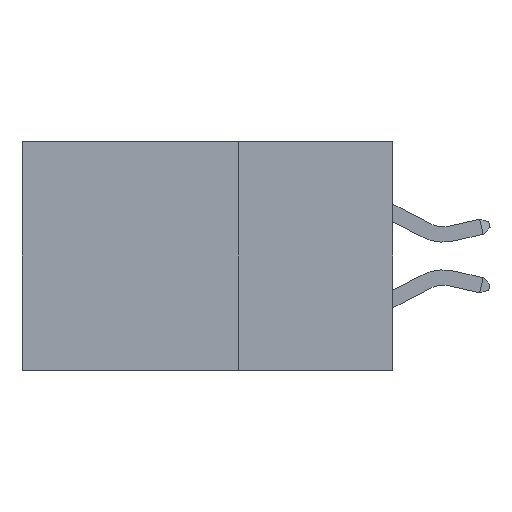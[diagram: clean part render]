
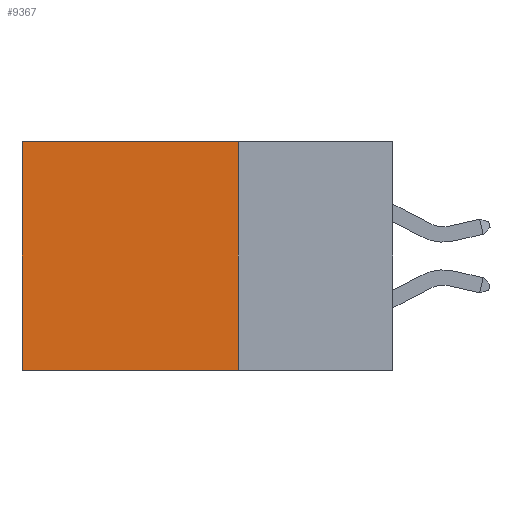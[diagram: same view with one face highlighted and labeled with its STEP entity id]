
A CAD part, left-side view. The second image highlights one B-rep face of the part: STEP entity #9367.
In plain terms, the highlighted planar face has unit normal (-1, 0, 0).
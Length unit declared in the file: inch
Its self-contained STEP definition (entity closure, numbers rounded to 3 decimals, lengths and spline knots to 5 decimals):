
#289 = DIRECTION ( 'NONE',  ( 1., 0., 0. ) ) ;
#455 = VECTOR ( 'NONE', #3845, 39.37008 ) ;
#1000 = CARTESIAN_POINT ( 'NONE',  ( 0.2875, 0.25, 0. ) ) ;
#2244 = FACE_OUTER_BOUND ( 'NONE', #4309, .T. ) ;
#2372 = ORIENTED_EDGE ( 'NONE', *, *, #8315, .T. ) ;
#3845 = DIRECTION ( 'NONE',  ( 0., 0., -1. ) ) ;
#4294 = VERTEX_POINT ( 'NONE', #1000 ) ;
#4309 = EDGE_LOOP ( 'NONE', ( #2372, #29610, #31092, #5243 ) ) ;
#5243 = ORIENTED_EDGE ( 'NONE', *, *, #23154, .T. ) ;
#5537 = DIRECTION ( 'NONE',  ( 0., 1., 0. ) ) ;
#6401 = CARTESIAN_POINT ( 'NONE',  ( 0.2875, 0.6, -0.37 ) ) ;
#6404 = VECTOR ( 'NONE', #21387, 39.37008 ) ;
#7165 = CARTESIAN_POINT ( 'NONE',  ( 0.2875, 0.25, 0. ) ) ;
#7296 = AXIS2_PLACEMENT_3D ( 'NONE', #7165, #289, #22230 ) ;
#8315 = EDGE_CURVE ( 'NONE', #25560, #11272, #31666, .T. ) ;
#8446 = CARTESIAN_POINT ( 'NONE',  ( 0.2875, 0.25, -0.37 ) ) ;
#8719 = LINE ( 'NONE', #23796, #14853 ) ;
#9367 = ADVANCED_FACE ( 'NONE', ( #2244 ), #22877, .F. ) ;
#11272 = VERTEX_POINT ( 'NONE', #6401 ) ;
#14264 = CARTESIAN_POINT ( 'NONE',  ( 0.2875, 0.6, 0. ) ) ;
#14853 = VECTOR ( 'NONE', #18219, 39.37008 ) ;
#15371 = EDGE_CURVE ( 'NONE', #4294, #20294, #21873, .T. ) ;
#16717 = VECTOR ( 'NONE', #5537, 39.37008 ) ;
#17970 = CARTESIAN_POINT ( 'NONE',  ( 0.2875, 0.25, 0. ) ) ;
#18219 = DIRECTION ( 'NONE',  ( 0., 1., 0. ) ) ;
#20294 = VERTEX_POINT ( 'NONE', #8446 ) ;
#21387 = DIRECTION ( 'NONE',  ( 0., 0., -1. ) ) ;
#21873 = LINE ( 'NONE', #29400, #6404 ) ;
#22230 = DIRECTION ( 'NONE',  ( 0., 0., -1. ) ) ;
#22877 = PLANE ( 'NONE',  #7296 ) ;
#23154 = EDGE_CURVE ( 'NONE', #4294, #25560, #25519, .T. ) ;
#23796 = CARTESIAN_POINT ( 'NONE',  ( 0.2875, 0.25, -0.37 ) ) ;
#24312 = CARTESIAN_POINT ( 'NONE',  ( 0.2875, 0.6, 0. ) ) ;
#25519 = LINE ( 'NONE', #17970, #16717 ) ;
#25560 = VERTEX_POINT ( 'NONE', #14264 ) ;
#29400 = CARTESIAN_POINT ( 'NONE',  ( 0.2875, 0.25, 0. ) ) ;
#29610 = ORIENTED_EDGE ( 'NONE', *, *, #30594, .F. ) ;
#30594 = EDGE_CURVE ( 'NONE', #20294, #11272, #8719, .T. ) ;
#31092 = ORIENTED_EDGE ( 'NONE', *, *, #15371, .F. ) ;
#31666 = LINE ( 'NONE', #24312, #455 ) ;
